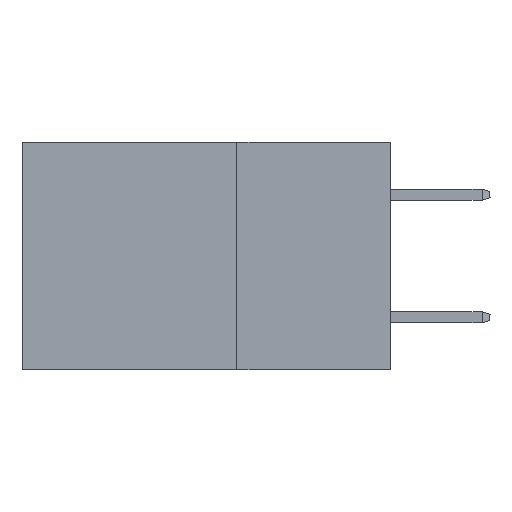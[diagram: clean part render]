
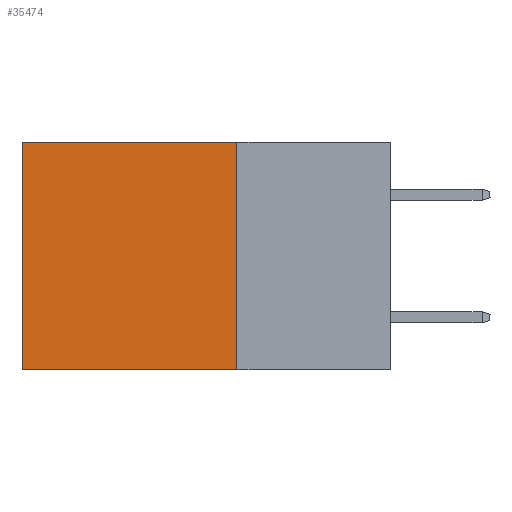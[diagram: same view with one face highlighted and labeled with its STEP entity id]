
A CAD part, left-side view. The second image highlights one B-rep face of the part: STEP entity #35474.
In plain terms, the highlighted planar face has unit normal (-1, 0, 0).
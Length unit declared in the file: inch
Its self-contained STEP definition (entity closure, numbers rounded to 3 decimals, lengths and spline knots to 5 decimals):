
#873 = DIRECTION ( 'NONE',  ( 1., 0., 0. ) ) ;
#1232 = CARTESIAN_POINT ( 'NONE',  ( 0.2875, 0.6, -0.37 ) ) ;
#2312 = FACE_OUTER_BOUND ( 'NONE', #29675, .T. ) ;
#2821 = DIRECTION ( 'NONE',  ( 0., 0., -1. ) ) ;
#5041 = CARTESIAN_POINT ( 'NONE',  ( 0.2875, 0.25, -0.37 ) ) ;
#8428 = VECTOR ( 'NONE', #10593, 39.37008 ) ;
#8550 = AXIS2_PLACEMENT_3D ( 'NONE', #15363, #873, #26386 ) ;
#9364 = VERTEX_POINT ( 'NONE', #22281 ) ;
#9891 = VECTOR ( 'NONE', #2821, 39.37008 ) ;
#10082 = LINE ( 'NONE', #11852, #28358 ) ;
#10150 = CARTESIAN_POINT ( 'NONE',  ( 0.2875, 0.6, 0. ) ) ;
#10593 = DIRECTION ( 'NONE',  ( 0., 0., -1. ) ) ;
#11852 = CARTESIAN_POINT ( 'NONE',  ( 0.2875, 0.25, -0.37 ) ) ;
#14885 = ORIENTED_EDGE ( 'NONE', *, *, #37529, .F. ) ;
#14961 = LINE ( 'NONE', #34693, #21277 ) ;
#15363 = CARTESIAN_POINT ( 'NONE',  ( 0.2875, 0.25, 0. ) ) ;
#18140 = LINE ( 'NONE', #25110, #8428 ) ;
#18585 = EDGE_CURVE ( 'NONE', #42388, #9364, #14961, .T. ) ;
#20796 = EDGE_CURVE ( 'NONE', #42388, #40463, #18140, .T. ) ;
#21277 = VECTOR ( 'NONE', #45719, 39.37008 ) ;
#22281 = CARTESIAN_POINT ( 'NONE',  ( 0.2875, 0.6, 0. ) ) ;
#22755 = PLANE ( 'NONE',  #8550 ) ;
#24895 = ORIENTED_EDGE ( 'NONE', *, *, #20796, .F. ) ;
#25110 = CARTESIAN_POINT ( 'NONE',  ( 0.2875, 0.25, 0. ) ) ;
#26386 = DIRECTION ( 'NONE',  ( 0., 0., -1. ) ) ;
#26760 = CARTESIAN_POINT ( 'NONE',  ( 0.2875, 0.25, 0. ) ) ;
#28358 = VECTOR ( 'NONE', #37398, 39.37008 ) ;
#29306 = LINE ( 'NONE', #10150, #9891 ) ;
#29375 = EDGE_CURVE ( 'NONE', #9364, #32581, #29306, .T. ) ;
#29675 = EDGE_LOOP ( 'NONE', ( #34637, #14885, #24895, #37573 ) ) ;
#32581 = VERTEX_POINT ( 'NONE', #1232 ) ;
#34637 = ORIENTED_EDGE ( 'NONE', *, *, #29375, .T. ) ;
#34693 = CARTESIAN_POINT ( 'NONE',  ( 0.2875, 0.25, 0. ) ) ;
#35474 = ADVANCED_FACE ( 'NONE', ( #2312 ), #22755, .F. ) ;
#37398 = DIRECTION ( 'NONE',  ( 0., 1., 0. ) ) ;
#37529 = EDGE_CURVE ( 'NONE', #40463, #32581, #10082, .T. ) ;
#37573 = ORIENTED_EDGE ( 'NONE', *, *, #18585, .T. ) ;
#40463 = VERTEX_POINT ( 'NONE', #5041 ) ;
#42388 = VERTEX_POINT ( 'NONE', #26760 ) ;
#45719 = DIRECTION ( 'NONE',  ( 0., 1., 0. ) ) ;
